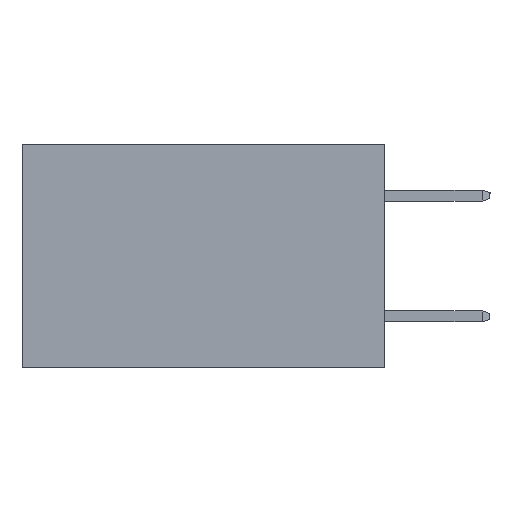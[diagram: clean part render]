
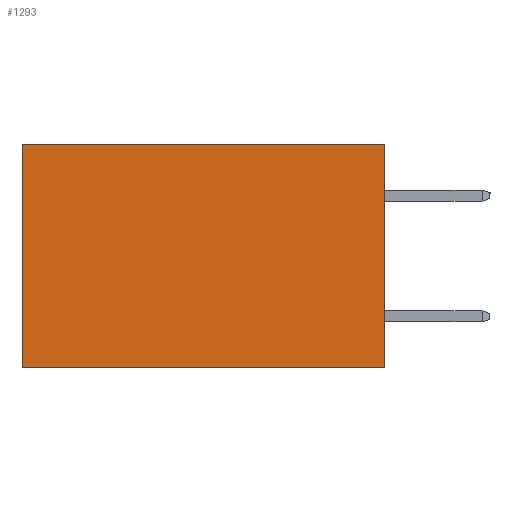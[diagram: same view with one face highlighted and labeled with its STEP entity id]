
A CAD part, left-side view. The second image highlights one B-rep face of the part: STEP entity #1293.
In plain terms, the highlighted planar face has unit normal (-1, 0, 0).
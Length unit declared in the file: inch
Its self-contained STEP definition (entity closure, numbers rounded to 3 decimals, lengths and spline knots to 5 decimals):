
#141 = VERTEX_POINT ( 'NONE', #424 ) ;
#368 = CARTESIAN_POINT ( 'NONE',  ( 0.2615, 0., -0.37 ) ) ;
#424 = CARTESIAN_POINT ( 'NONE',  ( 0.2615, 0.6, -0.37 ) ) ;
#651 = EDGE_CURVE ( 'NONE', #9031, #16647, #6546, .T. ) ;
#663 = DIRECTION ( 'NONE',  ( 1., 0., 0. ) ) ;
#1293 = ADVANCED_FACE ( 'NONE', ( #5276 ), #14703, .F. ) ;
#1945 = DIRECTION ( 'NONE',  ( 0., 0., -1. ) ) ;
#2181 = EDGE_CURVE ( 'NONE', #18882, #141, #19585, .T. ) ;
#3561 = DIRECTION ( 'NONE',  ( 0., 1., 0. ) ) ;
#5276 = FACE_OUTER_BOUND ( 'NONE', #12958, .T. ) ;
#6439 = EDGE_CURVE ( 'NONE', #16647, #141, #9818, .T. ) ;
#6546 = LINE ( 'NONE', #10000, #16743 ) ;
#7753 = VECTOR ( 'NONE', #1945, 39.37008 ) ;
#8341 = DIRECTION ( 'NONE',  ( 0., 0., -1. ) ) ;
#8476 = CARTESIAN_POINT ( 'NONE',  ( 0.2615, 0., -0.37 ) ) ;
#8525 = VECTOR ( 'NONE', #12891, 39.37008 ) ;
#8601 = VECTOR ( 'NONE', #9885, 39.37008 ) ;
#9031 = VERTEX_POINT ( 'NONE', #17617 ) ;
#9602 = CARTESIAN_POINT ( 'NONE',  ( 0.2615, 0., -0.37 ) ) ;
#9729 = CARTESIAN_POINT ( 'NONE',  ( 0.2615, 0.6, -0.37 ) ) ;
#9818 = LINE ( 'NONE', #9729, #7753 ) ;
#9885 = DIRECTION ( 'NONE',  ( 0., 1., 0. ) ) ;
#10000 = CARTESIAN_POINT ( 'NONE',  ( 0.2615, 0., 0. ) ) ;
#10433 = ORIENTED_EDGE ( 'NONE', *, *, #2181, .F. ) ;
#11558 = ORIENTED_EDGE ( 'NONE', *, *, #651, .T. ) ;
#12891 = DIRECTION ( 'NONE',  ( 0., 0., -1. ) ) ;
#12958 = EDGE_LOOP ( 'NONE', ( #15303, #10433, #13011, #11558 ) ) ;
#13011 = ORIENTED_EDGE ( 'NONE', *, *, #15530, .F. ) ;
#14703 = PLANE ( 'NONE',  #18381 ) ;
#14824 = CARTESIAN_POINT ( 'NONE',  ( 0.2615, 0., -0.37 ) ) ;
#15303 = ORIENTED_EDGE ( 'NONE', *, *, #6439, .T. ) ;
#15530 = EDGE_CURVE ( 'NONE', #9031, #18882, #17590, .T. ) ;
#16491 = CARTESIAN_POINT ( 'NONE',  ( 0.2615, 0.6, 0. ) ) ;
#16647 = VERTEX_POINT ( 'NONE', #16491 ) ;
#16743 = VECTOR ( 'NONE', #3561, 39.37008 ) ;
#17590 = LINE ( 'NONE', #9602, #8525 ) ;
#17617 = CARTESIAN_POINT ( 'NONE',  ( 0.2615, 0., 0. ) ) ;
#18381 = AXIS2_PLACEMENT_3D ( 'NONE', #368, #663, #8341 ) ;
#18882 = VERTEX_POINT ( 'NONE', #8476 ) ;
#19585 = LINE ( 'NONE', #14824, #8601 ) ;
